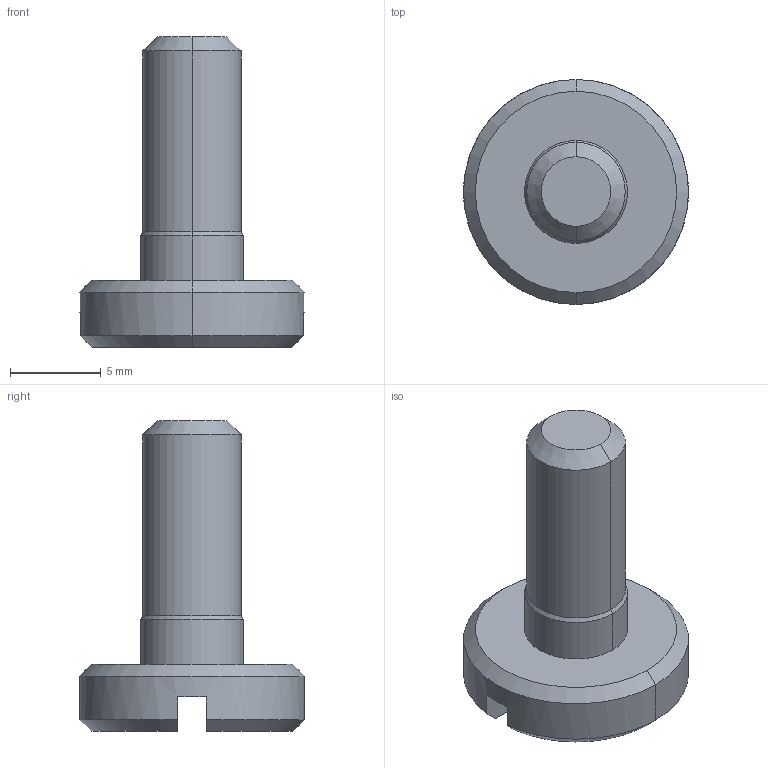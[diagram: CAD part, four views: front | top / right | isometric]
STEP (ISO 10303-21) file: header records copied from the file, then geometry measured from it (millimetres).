
FILE_DESCRIPTION (( 'STEP AP214' ), '1' );
FILE_NAME ('User Library-Telescopic Stock_Telescopic Stock Swivel Screw1.STEP', '2013-05-23T12:56:09', ( 'Asher' ), ( '' ), 'SwSTEP 2.0', 'SolidWorks 2013', '' );
FILE_SCHEMA (( 'AUTOMOTIVE_DESIGN' ));
Length unit declared in the file: millimetre
Products named in the file (1): User Library-Telescopic Stock_Telescopic Stock Swivel Screw1
Bounding box: 12.37 x 12.37 x 17.09 mm (x, y, z)
Volume: 699.2 mm3; surface area: 613.4 mm2
Topology: 1 solids, 1 shells, 22 faces, 48 edges, 29 vertices
Faces by surface type: cone 9, plane 7, cylinder 6
Entity records: 641 total; most frequent: DIRECTION 113, CARTESIAN_POINT 112, ORIENTED_EDGE 96, EDGE_CURVE 48, AXIS2_PLACEMENT_3D 46, VERTEX_POINT 29, EDGE_LOOP 23, CIRCLE 23
